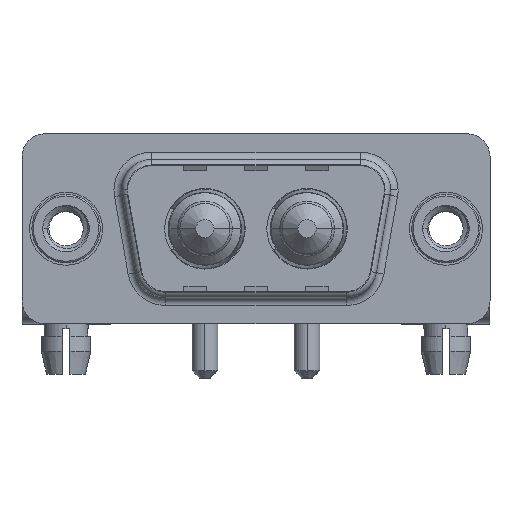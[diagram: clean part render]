
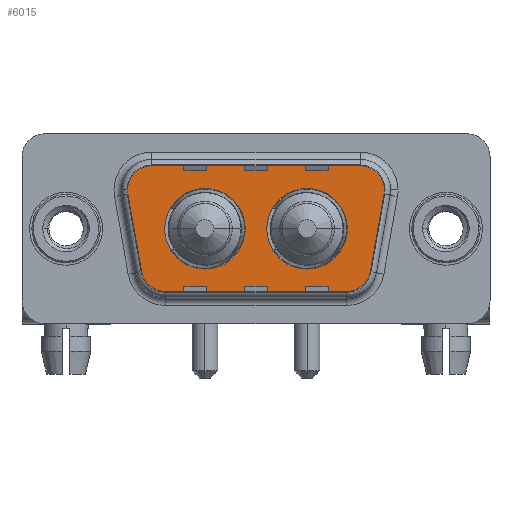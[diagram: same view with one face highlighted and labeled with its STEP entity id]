
A CAD part, top view. The second image highlights one B-rep face of the part: STEP entity #6015.
In plain terms, the highlighted planar face has unit normal (0, 0, 1).
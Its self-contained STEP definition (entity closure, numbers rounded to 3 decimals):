
#101 = CARTESIAN_POINT ( 'NONE',  ( 19.564, 2.9, 0. ) ) ;
#162 = DIRECTION ( 'NONE',  ( 0., 0., 1. ) ) ;
#190 = DIRECTION ( 'NONE',  ( 0.174, -0.985, 0. ) ) ;
#402 = VECTOR ( 'NONE', #190, 1000. ) ;
#414 = CARTESIAN_POINT ( 'NONE',  ( 3.466, 2.553, 0. ) ) ;
#594 = ORIENTED_EDGE ( 'NONE', *, *, #8923, .T. ) ;
#665 = AXIS2_PLACEMENT_3D ( 'NONE', #12908, #13073, #11921 ) ;
#974 = ORIENTED_EDGE ( 'NONE', *, *, #6135, .F. ) ;
#989 = VERTEX_POINT ( 'NONE', #2189 ) ;
#1146 = DIRECTION ( 'NONE',  ( -1., 0., 0. ) ) ;
#1148 = DIRECTION ( 'NONE',  ( 1., 0., 0. ) ) ;
#1160 = VERTEX_POINT ( 'NONE', #1275 ) ;
#1275 = CARTESIAN_POINT ( 'NONE',  ( 19.564, 4.9, 0. ) ) ;
#1308 = CARTESIAN_POINT ( 'NONE',  ( 6.459, -4.9, 0. ) ) ;
#1395 = LINE ( 'NONE', #5988, #402 ) ;
#1591 = ORIENTED_EDGE ( 'NONE', *, *, #9676, .F. ) ;
#1631 = AXIS2_PLACEMENT_3D ( 'NONE', #2889, #7648, #7573 ) ;
#1676 = CARTESIAN_POINT ( 'NONE',  ( 21.534, 2.553, 0. ) ) ;
#1712 = VECTOR ( 'NONE', #7987, 1000. ) ;
#1902 = ORIENTED_EDGE ( 'NONE', *, *, #6686, .F. ) ;
#2117 = DIRECTION ( 'NONE',  ( 0., 0., 1. ) ) ;
#2189 = CARTESIAN_POINT ( 'NONE',  ( 21.564, 2.9, 0. ) ) ;
#2357 = CARTESIAN_POINT ( 'NONE',  ( 15.86, 0., 0. ) ) ;
#2403 = AXIS2_PLACEMENT_3D ( 'NONE', #10175, #7882, #3191 ) ;
#2508 = CARTESIAN_POINT ( 'NONE',  ( 5.436, 4.9, 0. ) ) ;
#2741 = DIRECTION ( 'NONE',  ( 1., 0., 0. ) ) ;
#2791 = ORIENTED_EDGE ( 'NONE', *, *, #13818, .T. ) ;
#2818 = LINE ( 'NONE', #1676, #6735 ) ;
#2887 = CARTESIAN_POINT ( 'NONE',  ( 18.541, -2.9, 0. ) ) ;
#2889 = CARTESIAN_POINT ( 'NONE',  ( 19.564, 2.9, 0. ) ) ;
#2897 = CARTESIAN_POINT ( 'NONE',  ( 11.79, 0., 0. ) ) ;
#3041 = DIRECTION ( 'NONE',  ( 0., 0., 1. ) ) ;
#3070 = CIRCLE ( 'NONE', #10408, 2. ) ;
#3139 = CIRCLE ( 'NONE', #2403, 2. ) ;
#3191 = DIRECTION ( 'NONE',  ( -1., 0., 0. ) ) ;
#3230 = CIRCLE ( 'NONE', #7414, 2.65 ) ;
#3458 = VERTEX_POINT ( 'NONE', #7427 ) ;
#3559 = ORIENTED_EDGE ( 'NONE', *, *, #3936, .T. ) ;
#3874 = EDGE_LOOP ( 'NONE', ( #6190, #1902 ) ) ;
#3936 = EDGE_CURVE ( 'NONE', #4048, #11842, #1395, .T. ) ;
#3989 = VERTEX_POINT ( 'NONE', #4845 ) ;
#4024 = ORIENTED_EDGE ( 'NONE', *, *, #7428, .T. ) ;
#4048 = VERTEX_POINT ( 'NONE', #414 ) ;
#4364 = AXIS2_PLACEMENT_3D ( 'NONE', #13449, #12301, #13684 ) ;
#4372 = CARTESIAN_POINT ( 'NONE',  ( 20.511, -3.247, 0. ) ) ;
#4443 = CARTESIAN_POINT ( 'NONE',  ( 18.51, 0., 0. ) ) ;
#4619 = VERTEX_POINT ( 'NONE', #14658 ) ;
#4646 = EDGE_CURVE ( 'NONE', #4619, #989, #5786, .T. ) ;
#4845 = CARTESIAN_POINT ( 'NONE',  ( 6.459, -4.9, 0. ) ) ;
#5040 = AXIS2_PLACEMENT_3D ( 'NONE', #2887, #8793, #2741 ) ;
#5056 = CARTESIAN_POINT ( 'NONE',  ( 4.489, -3.247, 0. ) ) ;
#5302 = CIRCLE ( 'NONE', #665, 2.65 ) ;
#5786 = CIRCLE ( 'NONE', #1631, 2. ) ;
#5988 = CARTESIAN_POINT ( 'NONE',  ( 3.466, 2.553, 0. ) ) ;
#6015 = ADVANCED_FACE ( 'NONE', ( #14436, #13305, #14592 ), #14659, .T. ) ;
#6025 = EDGE_CURVE ( 'NONE', #11842, #3989, #3139, .T. ) ;
#6039 = CARTESIAN_POINT ( 'NONE',  ( 18.541, -4.9, 0. ) ) ;
#6135 = EDGE_CURVE ( 'NONE', #3458, #7739, #8540, .T. ) ;
#6190 = ORIENTED_EDGE ( 'NONE', *, *, #10705, .F. ) ;
#6211 = VERTEX_POINT ( 'NONE', #6039 ) ;
#6332 = VERTEX_POINT ( 'NONE', #8107 ) ;
#6686 = EDGE_CURVE ( 'NONE', #6332, #7362, #5302, .T. ) ;
#6721 = CARTESIAN_POINT ( 'NONE',  ( 9.14, 0., 0. ) ) ;
#6735 = VECTOR ( 'NONE', #7351, 1000. ) ;
#7351 = DIRECTION ( 'NONE',  ( 0.174, 0.985, 0. ) ) ;
#7362 = VERTEX_POINT ( 'NONE', #4443 ) ;
#7375 = EDGE_LOOP ( 'NONE', ( #14700, #2791, #8402, #594, #12418, #13014, #3559, #8152, #4024 ) ) ;
#7414 = AXIS2_PLACEMENT_3D ( 'NONE', #2357, #162, #1148 ) ;
#7427 = CARTESIAN_POINT ( 'NONE',  ( 6.49, 0., 0. ) ) ;
#7428 = EDGE_CURVE ( 'NONE', #3989, #6211, #11780, .T. ) ;
#7573 = DIRECTION ( 'NONE',  ( -1., 0., 0. ) ) ;
#7648 = DIRECTION ( 'NONE',  ( 0., 0., 1. ) ) ;
#7739 = VERTEX_POINT ( 'NONE', #2897 ) ;
#7852 = DIRECTION ( 'NONE',  ( 1., 0., 0. ) ) ;
#7868 = CIRCLE ( 'NONE', #12482, 2. ) ;
#7882 = DIRECTION ( 'NONE',  ( 0., 0., 1. ) ) ;
#7987 = DIRECTION ( 'NONE',  ( 1., 0., 0. ) ) ;
#8107 = CARTESIAN_POINT ( 'NONE',  ( 13.21, 0., 0. ) ) ;
#8122 = AXIS2_PLACEMENT_3D ( 'NONE', #12599, #2117, #11461 ) ;
#8152 = ORIENTED_EDGE ( 'NONE', *, *, #6025, .T. ) ;
#8270 = EDGE_CURVE ( 'NONE', #12579, #4048, #3070, .T. ) ;
#8402 = ORIENTED_EDGE ( 'NONE', *, *, #4646, .T. ) ;
#8540 = CIRCLE ( 'NONE', #13880, 2.65 ) ;
#8793 = DIRECTION ( 'NONE',  ( 0., 0., 1. ) ) ;
#8923 = EDGE_CURVE ( 'NONE', #989, #1160, #7868, .T. ) ;
#9069 = DIRECTION ( 'NONE',  ( 0., 0., 1. ) ) ;
#9253 = EDGE_CURVE ( 'NONE', #1160, #12579, #11316, .T. ) ;
#9426 = DIRECTION ( 'NONE',  ( 0., 0., 1. ) ) ;
#9676 = EDGE_CURVE ( 'NONE', #7739, #3458, #10303, .T. ) ;
#9923 = CIRCLE ( 'NONE', #5040, 2. ) ;
#10175 = CARTESIAN_POINT ( 'NONE',  ( 6.459, -2.9, 0. ) ) ;
#10303 = CIRCLE ( 'NONE', #8122, 2.65 ) ;
#10311 = DIRECTION ( 'NONE',  ( 1., 0., 0. ) ) ;
#10408 = AXIS2_PLACEMENT_3D ( 'NONE', #13657, #9069, #7852 ) ;
#10705 = EDGE_CURVE ( 'NONE', #7362, #6332, #3230, .T. ) ;
#11316 = LINE ( 'NONE', #2508, #12009 ) ;
#11461 = DIRECTION ( 'NONE',  ( 1., 0., 0. ) ) ;
#11613 = VERTEX_POINT ( 'NONE', #4372 ) ;
#11725 = CARTESIAN_POINT ( 'NONE',  ( 5.436, 4.9, 0. ) ) ;
#11780 = LINE ( 'NONE', #1308, #1712 ) ;
#11842 = VERTEX_POINT ( 'NONE', #5056 ) ;
#11921 = DIRECTION ( 'NONE',  ( 1., 0., 0. ) ) ;
#12009 = VECTOR ( 'NONE', #1146, 1000. ) ;
#12178 = EDGE_LOOP ( 'NONE', ( #1591, #974 ) ) ;
#12301 = DIRECTION ( 'NONE',  ( 0., 0., 1. ) ) ;
#12418 = ORIENTED_EDGE ( 'NONE', *, *, #9253, .T. ) ;
#12482 = AXIS2_PLACEMENT_3D ( 'NONE', #101, #9426, #14155 ) ;
#12579 = VERTEX_POINT ( 'NONE', #11725 ) ;
#12599 = CARTESIAN_POINT ( 'NONE',  ( 9.14, 0., 0. ) ) ;
#12908 = CARTESIAN_POINT ( 'NONE',  ( 15.86, 0., 0. ) ) ;
#13014 = ORIENTED_EDGE ( 'NONE', *, *, #8270, .T. ) ;
#13073 = DIRECTION ( 'NONE',  ( 0., 0., 1. ) ) ;
#13305 = FACE_BOUND ( 'NONE', #12178, .T. ) ;
#13449 = CARTESIAN_POINT ( 'NONE',  ( 18.541, -2.9, 0. ) ) ;
#13657 = CARTESIAN_POINT ( 'NONE',  ( 5.436, 2.9, 0. ) ) ;
#13684 = DIRECTION ( 'NONE',  ( 1., 0., 0. ) ) ;
#13818 = EDGE_CURVE ( 'NONE', #11613, #4619, #2818, .T. ) ;
#13839 = EDGE_CURVE ( 'NONE', #6211, #11613, #9923, .T. ) ;
#13880 = AXIS2_PLACEMENT_3D ( 'NONE', #6721, #3041, #10311 ) ;
#14155 = DIRECTION ( 'NONE',  ( -1., 0., 0. ) ) ;
#14436 = FACE_BOUND ( 'NONE', #3874, .T. ) ;
#14592 = FACE_OUTER_BOUND ( 'NONE', #7375, .T. ) ;
#14658 = CARTESIAN_POINT ( 'NONE',  ( 21.534, 2.553, 0. ) ) ;
#14659 = PLANE ( 'NONE',  #4364 ) ;
#14700 = ORIENTED_EDGE ( 'NONE', *, *, #13839, .T. ) ;
